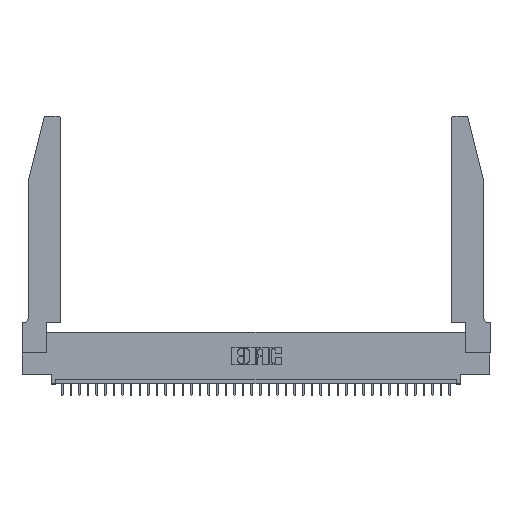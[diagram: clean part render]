
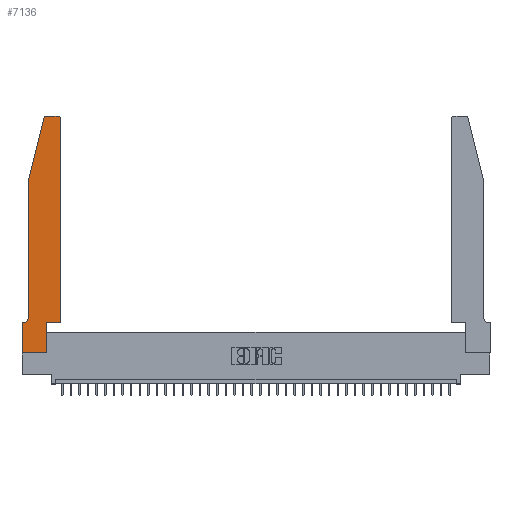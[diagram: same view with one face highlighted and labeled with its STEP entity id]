
A CAD part, top view. The second image highlights one B-rep face of the part: STEP entity #7136.
In plain terms, the highlighted planar face has unit normal (0, 0, 1).
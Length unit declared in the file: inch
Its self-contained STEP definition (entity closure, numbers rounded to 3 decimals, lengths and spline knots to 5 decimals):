
#117 = VECTOR ( 'NONE', #12181, 39.37008 ) ;
#148 = VECTOR ( 'NONE', #18252, 39.37008 ) ;
#209 = EDGE_CURVE ( 'NONE', #10000, #33814, #25744, .T. ) ;
#1729 = LINE ( 'NONE', #17102, #21222 ) ;
#2208 = CARTESIAN_POINT ( 'NONE',  ( 0.4205, 2.75, 0.37 ) ) ;
#2425 = CIRCLE ( 'NONE', #34642, 0.03 ) ;
#2826 = VERTEX_POINT ( 'NONE', #24737 ) ;
#3296 = CARTESIAN_POINT ( 'NONE',  ( 0.4505, 0.35, 0.37 ) ) ;
#3617 = CARTESIAN_POINT ( 'NONE',  ( 0.0755, 0.42, 0.37 ) ) ;
#4022 = LINE ( 'NONE', #25151, #31783 ) ;
#4500 = CARTESIAN_POINT ( 'NONE',  ( 0.4505, 2.72, 0.37 ) ) ;
#4814 = LINE ( 'NONE', #37629, #18643 ) ;
#5224 = VERTEX_POINT ( 'NONE', #29951 ) ;
#5277 = ORIENTED_EDGE ( 'NONE', *, *, #38988, .T. ) ;
#5563 = CARTESIAN_POINT ( 'NONE',  ( 0., 0., 0.37 ) ) ;
#5883 = CARTESIAN_POINT ( 'NONE',  ( 0.284, 2.75, 0.37 ) ) ;
#6475 = CARTESIAN_POINT ( 'NONE',  ( 0.0755, 2., 0.37 ) ) ;
#7136 = ADVANCED_FACE ( 'NONE', ( #13848 ), #10508, .T. ) ;
#7190 = DIRECTION ( 'NONE',  ( 0., 1., 0. ) ) ;
#7747 = CARTESIAN_POINT ( 'NONE',  ( 0., 0.35, 0.37 ) ) ;
#8127 = VERTEX_POINT ( 'NONE', #23270 ) ;
#8184 = EDGE_CURVE ( 'NONE', #31113, #2826, #17512, .T. ) ;
#8341 = ORIENTED_EDGE ( 'NONE', *, *, #37745, .T. ) ;
#8652 = VERTEX_POINT ( 'NONE', #21183 ) ;
#8724 = CARTESIAN_POINT ( 'NONE',  ( 0.4205, 2.72, 0.37 ) ) ;
#8951 = EDGE_CURVE ( 'NONE', #25570, #10000, #11982, .T. ) ;
#10000 = VERTEX_POINT ( 'NONE', #3617 ) ;
#10205 = ORIENTED_EDGE ( 'NONE', *, *, #27202, .T. ) ;
#10334 = VECTOR ( 'NONE', #17599, 39.37008 ) ;
#10506 = AXIS2_PLACEMENT_3D ( 'NONE', #22754, #38172, #25707 ) ;
#10508 = PLANE ( 'NONE',  #22821 ) ;
#10976 = DIRECTION ( 'NONE',  ( -0.239, -0.971, 0. ) ) ;
#11229 = EDGE_CURVE ( 'NONE', #5224, #31113, #4022, .T. ) ;
#11505 = EDGE_CURVE ( 'NONE', #8127, #5224, #26684, .T. ) ;
#11888 = DIRECTION ( 'NONE',  ( -1., 0., 0. ) ) ;
#11982 = LINE ( 'NONE', #6475, #117 ) ;
#12181 = DIRECTION ( 'NONE',  ( 0., -1., 0. ) ) ;
#13359 = LINE ( 'NONE', #31758, #30302 ) ;
#13848 = FACE_OUTER_BOUND ( 'NONE', #22081, .T. ) ;
#14242 = EDGE_CURVE ( 'NONE', #8652, #25570, #1729, .T. ) ;
#15361 = VERTEX_POINT ( 'NONE', #4500 ) ;
#16047 = DIRECTION ( 'NONE',  ( 1., 0., 0. ) ) ;
#16823 = DIRECTION ( 'NONE',  ( 1., 0., 0. ) ) ;
#16847 = ORIENTED_EDGE ( 'NONE', *, *, #209, .T. ) ;
#17102 = CARTESIAN_POINT ( 'NONE',  ( 0.0755, 2., 0.37 ) ) ;
#17512 = LINE ( 'NONE', #29382, #148 ) ;
#17599 = DIRECTION ( 'NONE',  ( 0., -1., 0. ) ) ;
#18252 = DIRECTION ( 'NONE',  ( 0., 1., 0. ) ) ;
#18643 = VECTOR ( 'NONE', #28715, 39.37008 ) ;
#19595 = ORIENTED_EDGE ( 'NONE', *, *, #11505, .T. ) ;
#19870 = VERTEX_POINT ( 'NONE', #3296 ) ;
#20662 = VECTOR ( 'NONE', #7190, 39.37008 ) ;
#21183 = CARTESIAN_POINT ( 'NONE',  ( 0.25487, 2.72718, 0.37 ) ) ;
#21191 = DIRECTION ( 'NONE',  ( 0., 0., -1. ) ) ;
#21222 = VECTOR ( 'NONE', #10976, 39.37008 ) ;
#21442 = ORIENTED_EDGE ( 'NONE', *, *, #14242, .T. ) ;
#22081 = EDGE_LOOP ( 'NONE', ( #10205, #34736, #21442, #29498, #16847, #25370, #19595, #27362, #35246, #29164, #8341, #5277 ) ) ;
#22221 = LINE ( 'NONE', #34295, #20662 ) ;
#22480 = DIRECTION ( 'NONE',  ( -1., 0., 0. ) ) ;
#22754 = CARTESIAN_POINT ( 'NONE',  ( 0.284, 2.72, 0.37 ) ) ;
#22821 = AXIS2_PLACEMENT_3D ( 'NONE', #7747, #28698, #16823 ) ;
#23176 = DIRECTION ( 'NONE',  ( 1., 0., 0. ) ) ;
#23270 = CARTESIAN_POINT ( 'NONE',  ( 0., 0.35, 0.37 ) ) ;
#23760 = DIRECTION ( 'NONE',  ( 0., 0., 1. ) ) ;
#23956 = CARTESIAN_POINT ( 'NONE',  ( 0.0055, 0.35, 0.37 ) ) ;
#24308 = VERTEX_POINT ( 'NONE', #2208 ) ;
#24376 = CARTESIAN_POINT ( 'NONE',  ( 0.2605, 2.75, 0.37 ) ) ;
#24737 = CARTESIAN_POINT ( 'NONE',  ( 0.2865, 0.35, 0.37 ) ) ;
#25151 = CARTESIAN_POINT ( 'NONE',  ( 0., 0., 0.37 ) ) ;
#25294 = EDGE_CURVE ( 'NONE', #33814, #8127, #13359, .T. ) ;
#25370 = ORIENTED_EDGE ( 'NONE', *, *, #25294, .T. ) ;
#25570 = VERTEX_POINT ( 'NONE', #30354 ) ;
#25707 = DIRECTION ( 'NONE',  ( 1., 0., 0. ) ) ;
#25744 = CIRCLE ( 'NONE', #29523, 0.07 ) ;
#26684 = LINE ( 'NONE', #5563, #10334 ) ;
#27202 = EDGE_CURVE ( 'NONE', #24308, #34600, #36651, .T. ) ;
#27362 = ORIENTED_EDGE ( 'NONE', *, *, #11229, .T. ) ;
#27551 = CIRCLE ( 'NONE', #10506, 0.03 ) ;
#28698 = DIRECTION ( 'NONE',  ( 0., 0., 1. ) ) ;
#28715 = DIRECTION ( 'NONE',  ( 1., 0., 0. ) ) ;
#29164 = ORIENTED_EDGE ( 'NONE', *, *, #33685, .T. ) ;
#29382 = CARTESIAN_POINT ( 'NONE',  ( 0.2865, 0.35, 0.37 ) ) ;
#29498 = ORIENTED_EDGE ( 'NONE', *, *, #8951, .T. ) ;
#29523 = AXIS2_PLACEMENT_3D ( 'NONE', #35659, #21191, #11888 ) ;
#29951 = CARTESIAN_POINT ( 'NONE',  ( 0., 0., 0.37 ) ) ;
#30302 = VECTOR ( 'NONE', #22480, 39.37008 ) ;
#30354 = CARTESIAN_POINT ( 'NONE',  ( 0.0755, 2., 0.37 ) ) ;
#30905 = DIRECTION ( 'NONE',  ( -1., 0., 0. ) ) ;
#31113 = VERTEX_POINT ( 'NONE', #33624 ) ;
#31758 = CARTESIAN_POINT ( 'NONE',  ( 0.0755, 0.35, 0.37 ) ) ;
#31783 = VECTOR ( 'NONE', #16047, 39.37008 ) ;
#33624 = CARTESIAN_POINT ( 'NONE',  ( 0.2865, 0., 0.37 ) ) ;
#33685 = EDGE_CURVE ( 'NONE', #2826, #19870, #4814, .T. ) ;
#33814 = VERTEX_POINT ( 'NONE', #23956 ) ;
#34295 = CARTESIAN_POINT ( 'NONE',  ( 0.4505, 0.35, 0.37 ) ) ;
#34600 = VERTEX_POINT ( 'NONE', #5883 ) ;
#34642 = AXIS2_PLACEMENT_3D ( 'NONE', #8724, #23760, #23176 ) ;
#34736 = ORIENTED_EDGE ( 'NONE', *, *, #35450, .T. ) ;
#35246 = ORIENTED_EDGE ( 'NONE', *, *, #8184, .T. ) ;
#35450 = EDGE_CURVE ( 'NONE', #34600, #8652, #27551, .T. ) ;
#35659 = CARTESIAN_POINT ( 'NONE',  ( 0.0055, 0.42, 0.37 ) ) ;
#36126 = VECTOR ( 'NONE', #30905, 39.37008 ) ;
#36651 = LINE ( 'NONE', #24376, #36126 ) ;
#37629 = CARTESIAN_POINT ( 'NONE',  ( 0.4505, 0.35, 0.37 ) ) ;
#37745 = EDGE_CURVE ( 'NONE', #19870, #15361, #22221, .T. ) ;
#38172 = DIRECTION ( 'NONE',  ( 0., 0., 1. ) ) ;
#38988 = EDGE_CURVE ( 'NONE', #15361, #24308, #2425, .T. ) ;
